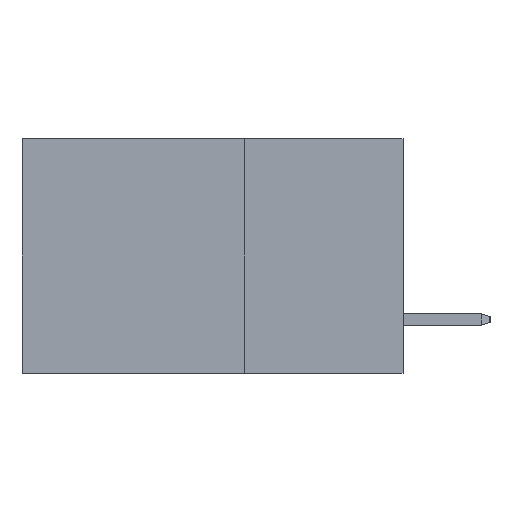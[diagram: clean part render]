
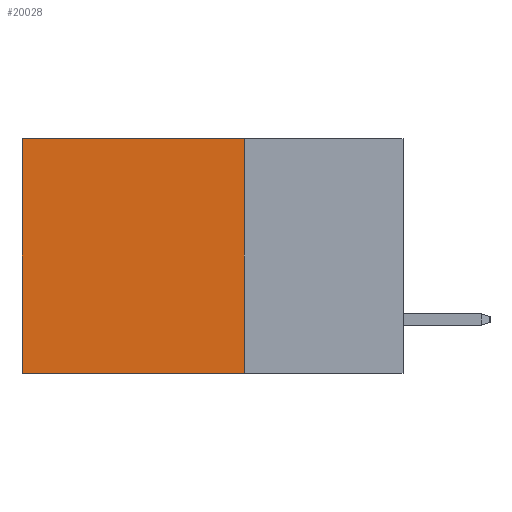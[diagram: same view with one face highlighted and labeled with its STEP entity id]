
A CAD part, left-side view. The second image highlights one B-rep face of the part: STEP entity #20028.
In plain terms, the highlighted planar face has unit normal (-1, 0, 0).
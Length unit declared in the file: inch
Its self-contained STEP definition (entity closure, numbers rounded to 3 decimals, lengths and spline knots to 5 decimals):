
#983 = ORIENTED_EDGE ( 'NONE', *, *, #7653, .T. ) ;
#1038 = AXIS2_PLACEMENT_3D ( 'NONE', #11289, #8312, #1793 ) ;
#1150 = EDGE_CURVE ( 'NONE', #10373, #15969, #16267, .T. ) ;
#1793 = DIRECTION ( 'NONE',  ( 0., 0., -1. ) ) ;
#2384 = LINE ( 'NONE', #9233, #17946 ) ;
#2545 = VERTEX_POINT ( 'NONE', #13690 ) ;
#3057 = LINE ( 'NONE', #16008, #10866 ) ;
#4447 = FACE_OUTER_BOUND ( 'NONE', #17553, .T. ) ;
#5521 = VERTEX_POINT ( 'NONE', #7677 ) ;
#5971 = LINE ( 'NONE', #17290, #7642 ) ;
#7642 = VECTOR ( 'NONE', #7680, 39.37008 ) ;
#7653 = EDGE_CURVE ( 'NONE', #5521, #10373, #5971, .T. ) ;
#7677 = CARTESIAN_POINT ( 'NONE',  ( 0.2875, 0.25, 0. ) ) ;
#7680 = DIRECTION ( 'NONE',  ( 0., 1., 0. ) ) ;
#7714 = DIRECTION ( 'NONE',  ( 0., 0., -1. ) ) ;
#8312 = DIRECTION ( 'NONE',  ( 1., 0., 0. ) ) ;
#9233 = CARTESIAN_POINT ( 'NONE',  ( 0.2875, 0.25, -0.37 ) ) ;
#9850 = EDGE_CURVE ( 'NONE', #2545, #15969, #2384, .T. ) ;
#10373 = VERTEX_POINT ( 'NONE', #19467 ) ;
#10866 = VECTOR ( 'NONE', #14296, 39.37008 ) ;
#10970 = PLANE ( 'NONE',  #1038 ) ;
#11289 = CARTESIAN_POINT ( 'NONE',  ( 0.2875, 0.25, 0. ) ) ;
#12610 = CARTESIAN_POINT ( 'NONE',  ( 0.2875, 0.6, 0. ) ) ;
#13690 = CARTESIAN_POINT ( 'NONE',  ( 0.2875, 0.25, -0.37 ) ) ;
#14296 = DIRECTION ( 'NONE',  ( 0., 0., -1. ) ) ;
#14636 = EDGE_CURVE ( 'NONE', #5521, #2545, #3057, .T. ) ;
#14710 = ORIENTED_EDGE ( 'NONE', *, *, #9850, .F. ) ;
#15745 = DIRECTION ( 'NONE',  ( 0., 1., 0. ) ) ;
#15969 = VERTEX_POINT ( 'NONE', #17872 ) ;
#16008 = CARTESIAN_POINT ( 'NONE',  ( 0.2875, 0.25, 0. ) ) ;
#16267 = LINE ( 'NONE', #12610, #20478 ) ;
#17290 = CARTESIAN_POINT ( 'NONE',  ( 0.2875, 0.25, 0. ) ) ;
#17553 = EDGE_LOOP ( 'NONE', ( #18380, #14710, #18607, #983 ) ) ;
#17872 = CARTESIAN_POINT ( 'NONE',  ( 0.2875, 0.6, -0.37 ) ) ;
#17946 = VECTOR ( 'NONE', #15745, 39.37008 ) ;
#18380 = ORIENTED_EDGE ( 'NONE', *, *, #1150, .T. ) ;
#18607 = ORIENTED_EDGE ( 'NONE', *, *, #14636, .F. ) ;
#19467 = CARTESIAN_POINT ( 'NONE',  ( 0.2875, 0.6, 0. ) ) ;
#20028 = ADVANCED_FACE ( 'NONE', ( #4447 ), #10970, .F. ) ;
#20478 = VECTOR ( 'NONE', #7714, 39.37008 ) ;
